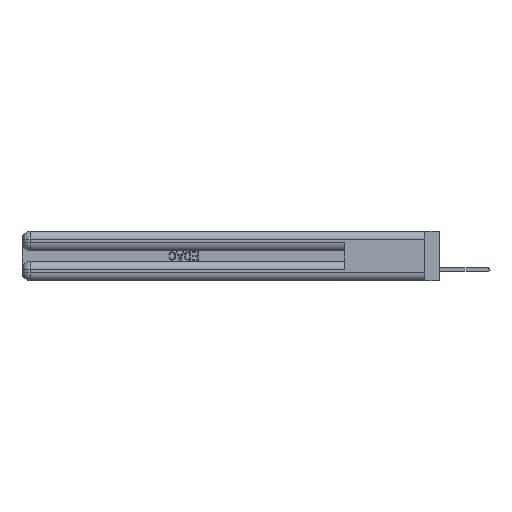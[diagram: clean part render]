
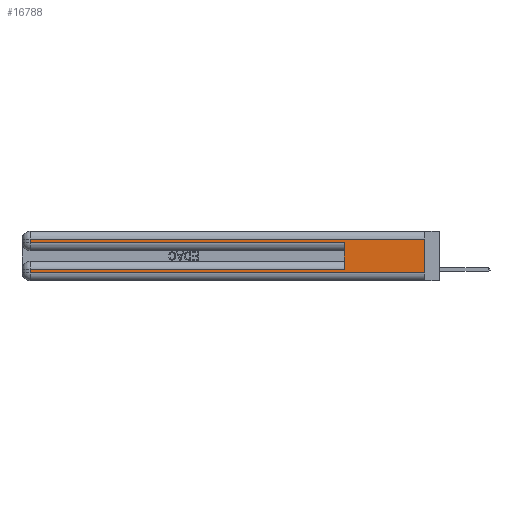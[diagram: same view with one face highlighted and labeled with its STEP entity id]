
A CAD part, left-side view. The second image highlights one B-rep face of the part: STEP entity #16788.
In plain terms, the highlighted planar face has unit normal (-1, 0, 0).
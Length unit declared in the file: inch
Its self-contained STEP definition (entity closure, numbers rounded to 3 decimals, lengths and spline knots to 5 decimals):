
#776 = DIRECTION ( 'NONE',  ( 0., 0., -1. ) ) ;
#1313 = LINE ( 'NONE', #13666, #42243 ) ;
#2259 = LINE ( 'NONE', #6658, #22000 ) ;
#3404 = CARTESIAN_POINT ( 'NONE',  ( 0., 2.94, 0.31 ) ) ;
#4602 = FACE_OUTER_BOUND ( 'NONE', #9884, .T. ) ;
#4724 = CARTESIAN_POINT ( 'NONE',  ( 0., 0., 0.37 ) ) ;
#5216 = EDGE_CURVE ( 'NONE', #36149, #33134, #16172, .T. ) ;
#5368 = VECTOR ( 'NONE', #38804, 39.37008 ) ;
#5704 = VECTOR ( 'NONE', #31273, 39.37008 ) ;
#5878 = ORIENTED_EDGE ( 'NONE', *, *, #5216, .F. ) ;
#6658 = CARTESIAN_POINT ( 'NONE',  ( 0., 0., 0.285 ) ) ;
#6795 = VERTEX_POINT ( 'NONE', #48430 ) ;
#7290 = VECTOR ( 'NONE', #13835, 39.37008 ) ;
#7871 = ORIENTED_EDGE ( 'NONE', *, *, #15606, .T. ) ;
#7974 = ORIENTED_EDGE ( 'NONE', *, *, #11190, .T. ) ;
#9360 = VERTEX_POINT ( 'NONE', #49970 ) ;
#9884 = EDGE_LOOP ( 'NONE', ( #5878, #18971, #7974, #35172, #10500, #7871, #19538, #50809 ) ) ;
#10500 = ORIENTED_EDGE ( 'NONE', *, *, #15140, .F. ) ;
#10713 = CARTESIAN_POINT ( 'NONE',  ( 0., 0.6, 0.085 ) ) ;
#10988 = CARTESIAN_POINT ( 'NONE',  ( 0., 0., 0.31 ) ) ;
#11190 = EDGE_CURVE ( 'NONE', #50949, #6795, #25180, .T. ) ;
#13666 = CARTESIAN_POINT ( 'NONE',  ( 0., 2.94, 0.37 ) ) ;
#13835 = DIRECTION ( 'NONE',  ( 0., 0., 1. ) ) ;
#14372 = CARTESIAN_POINT ( 'NONE',  ( 0., 0., 0.085 ) ) ;
#14820 = DIRECTION ( 'NONE',  ( 0., 0., -1. ) ) ;
#15140 = EDGE_CURVE ( 'NONE', #19789, #9360, #30844, .T. ) ;
#15442 = CARTESIAN_POINT ( 'NONE',  ( 0., 0., 0.37 ) ) ;
#15606 = EDGE_CURVE ( 'NONE', #19789, #36108, #15875, .T. ) ;
#15875 = LINE ( 'NONE', #14372, #35803 ) ;
#16172 = LINE ( 'NONE', #15442, #5704 ) ;
#16788 = ADVANCED_FACE ( 'NONE', ( #4602 ), #43885, .F. ) ;
#18609 = CARTESIAN_POINT ( 'NONE',  ( 0., 2.94, 0.37 ) ) ;
#18971 = ORIENTED_EDGE ( 'NONE', *, *, #33591, .T. ) ;
#19538 = ORIENTED_EDGE ( 'NONE', *, *, #42714, .T. ) ;
#19789 = VERTEX_POINT ( 'NONE', #10713 ) ;
#22000 = VECTOR ( 'NONE', #46276, 39.37008 ) ;
#22513 = DIRECTION ( 'NONE',  ( 0., 1., 0. ) ) ;
#23428 = VECTOR ( 'NONE', #34907, 39.37008 ) ;
#24900 = CARTESIAN_POINT ( 'NONE',  ( 0., 2.94, 0.085 ) ) ;
#25180 = LINE ( 'NONE', #18609, #37652 ) ;
#27683 = LINE ( 'NONE', #10988, #5368 ) ;
#29959 = AXIS2_PLACEMENT_3D ( 'NONE', #4724, #40627, #776 ) ;
#30844 = LINE ( 'NONE', #38028, #7290 ) ;
#31273 = DIRECTION ( 'NONE',  ( 0., 0., -1. ) ) ;
#33134 = VERTEX_POINT ( 'NONE', #47600 ) ;
#33591 = EDGE_CURVE ( 'NONE', #36149, #50949, #27683, .T. ) ;
#33925 = CARTESIAN_POINT ( 'NONE',  ( 0., 2.94, 0.06 ) ) ;
#34907 = DIRECTION ( 'NONE',  ( 0., -1., 0. ) ) ;
#35158 = VERTEX_POINT ( 'NONE', #33925 ) ;
#35172 = ORIENTED_EDGE ( 'NONE', *, *, #49020, .T. ) ;
#35184 = CARTESIAN_POINT ( 'NONE',  ( 0., 0., 0.31 ) ) ;
#35266 = LINE ( 'NONE', #47149, #23428 ) ;
#35803 = VECTOR ( 'NONE', #22513, 39.37008 ) ;
#36108 = VERTEX_POINT ( 'NONE', #24900 ) ;
#36149 = VERTEX_POINT ( 'NONE', #35184 ) ;
#37652 = VECTOR ( 'NONE', #14820, 39.37008 ) ;
#38028 = CARTESIAN_POINT ( 'NONE',  ( 0., 0.6, 0.145 ) ) ;
#38804 = DIRECTION ( 'NONE',  ( 0., 1., 0. ) ) ;
#40627 = DIRECTION ( 'NONE',  ( 1., 0., 0. ) ) ;
#42243 = VECTOR ( 'NONE', #45363, 39.37008 ) ;
#42714 = EDGE_CURVE ( 'NONE', #36108, #35158, #1313, .T. ) ;
#43885 = PLANE ( 'NONE',  #29959 ) ;
#45363 = DIRECTION ( 'NONE',  ( 0., 0., -1. ) ) ;
#46276 = DIRECTION ( 'NONE',  ( 0., -1., 0. ) ) ;
#46523 = EDGE_CURVE ( 'NONE', #35158, #33134, #35266, .T. ) ;
#47149 = CARTESIAN_POINT ( 'NONE',  ( 0., 0., 0.06 ) ) ;
#47600 = CARTESIAN_POINT ( 'NONE',  ( 0., 0., 0.06 ) ) ;
#48430 = CARTESIAN_POINT ( 'NONE',  ( 0., 2.94, 0.285 ) ) ;
#49020 = EDGE_CURVE ( 'NONE', #6795, #9360, #2259, .T. ) ;
#49970 = CARTESIAN_POINT ( 'NONE',  ( 0., 0.6, 0.285 ) ) ;
#50809 = ORIENTED_EDGE ( 'NONE', *, *, #46523, .T. ) ;
#50949 = VERTEX_POINT ( 'NONE', #3404 ) ;
